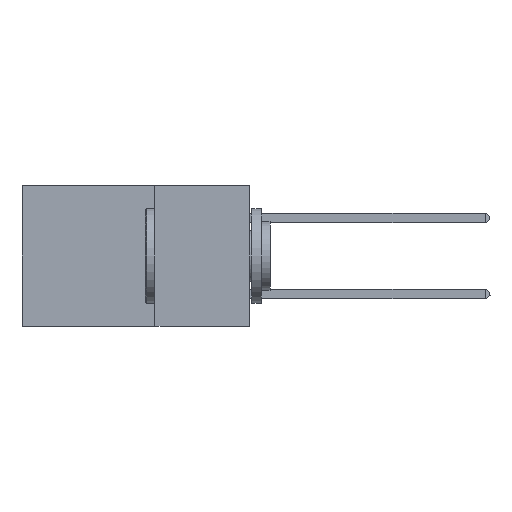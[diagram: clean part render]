
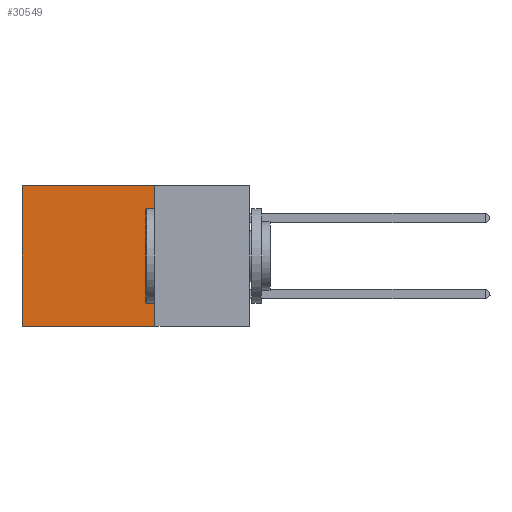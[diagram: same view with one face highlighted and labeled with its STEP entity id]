
A CAD part, left-side view. The second image highlights one B-rep face of the part: STEP entity #30549.
In plain terms, the highlighted planar face has unit normal (-1, 0, 0).
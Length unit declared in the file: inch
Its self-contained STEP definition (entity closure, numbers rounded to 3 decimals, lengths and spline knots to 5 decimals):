
#2384 = EDGE_CURVE ( 'NONE', #3620, #27322, #9553, .T. ) ;
#2803 = ORIENTED_EDGE ( 'NONE', *, *, #2384, .T. ) ;
#3620 = VERTEX_POINT ( 'NONE', #36179 ) ;
#4513 = EDGE_CURVE ( 'NONE', #26771, #27322, #31384, .T. ) ;
#4712 = CARTESIAN_POINT ( 'NONE',  ( 0.2875, 0.6, 0. ) ) ;
#5686 = CARTESIAN_POINT ( 'NONE',  ( 0.2875, 0.25, 0. ) ) ;
#5875 = VECTOR ( 'NONE', #28198, 39.37008 ) ;
#6197 = EDGE_LOOP ( 'NONE', ( #2803, #25078, #23900, #10866 ) ) ;
#6550 = CARTESIAN_POINT ( 'NONE',  ( 0.2875, 0.25, 0. ) ) ;
#6573 = PLANE ( 'NONE',  #17678 ) ;
#7564 = CARTESIAN_POINT ( 'NONE',  ( 0.2875, 0.25, -0.37 ) ) ;
#8527 = VECTOR ( 'NONE', #23890, 39.37008 ) ;
#8809 = CARTESIAN_POINT ( 'NONE',  ( 0.2875, 0.25, 0. ) ) ;
#9553 = LINE ( 'NONE', #4712, #8527 ) ;
#9820 = DIRECTION ( 'NONE',  ( 0., 0., -1. ) ) ;
#10866 = ORIENTED_EDGE ( 'NONE', *, *, #12719, .T. ) ;
#12216 = CARTESIAN_POINT ( 'NONE',  ( 0.2875, 0.25, -0.37 ) ) ;
#12719 = EDGE_CURVE ( 'NONE', #39006, #3620, #17165, .T. ) ;
#14196 = VECTOR ( 'NONE', #38381, 39.37008 ) ;
#17165 = LINE ( 'NONE', #6550, #14196 ) ;
#17678 = AXIS2_PLACEMENT_3D ( 'NONE', #22557, #28942, #9820 ) ;
#19933 = EDGE_CURVE ( 'NONE', #39006, #26771, #38415, .T. ) ;
#22557 = CARTESIAN_POINT ( 'NONE',  ( 0.2875, 0.25, 0. ) ) ;
#23890 = DIRECTION ( 'NONE',  ( 0., 0., -1. ) ) ;
#23900 = ORIENTED_EDGE ( 'NONE', *, *, #19933, .F. ) ;
#25078 = ORIENTED_EDGE ( 'NONE', *, *, #4513, .F. ) ;
#26137 = CARTESIAN_POINT ( 'NONE',  ( 0.2875, 0.6, -0.37 ) ) ;
#26771 = VERTEX_POINT ( 'NONE', #7564 ) ;
#27322 = VERTEX_POINT ( 'NONE', #26137 ) ;
#28198 = DIRECTION ( 'NONE',  ( 0., 1., 0. ) ) ;
#28942 = DIRECTION ( 'NONE',  ( 1., 0., 0. ) ) ;
#29949 = VECTOR ( 'NONE', #34360, 39.37008 ) ;
#30549 = ADVANCED_FACE ( 'NONE', ( #35095 ), #6573, .F. ) ;
#31384 = LINE ( 'NONE', #12216, #5875 ) ;
#34360 = DIRECTION ( 'NONE',  ( 0., 0., -1. ) ) ;
#35095 = FACE_OUTER_BOUND ( 'NONE', #6197, .T. ) ;
#36179 = CARTESIAN_POINT ( 'NONE',  ( 0.2875, 0.6, 0. ) ) ;
#38381 = DIRECTION ( 'NONE',  ( 0., 1., 0. ) ) ;
#38415 = LINE ( 'NONE', #5686, #29949 ) ;
#39006 = VERTEX_POINT ( 'NONE', #8809 ) ;
